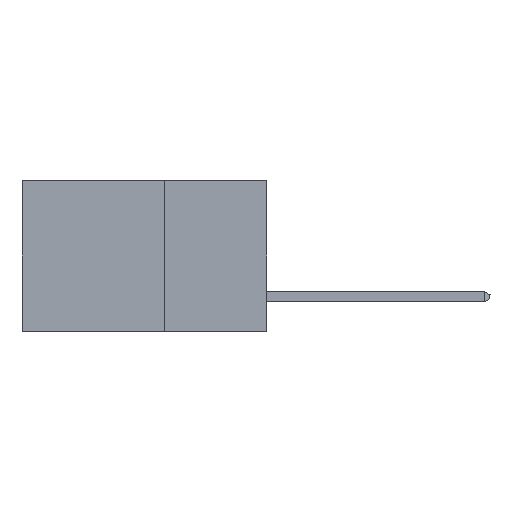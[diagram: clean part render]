
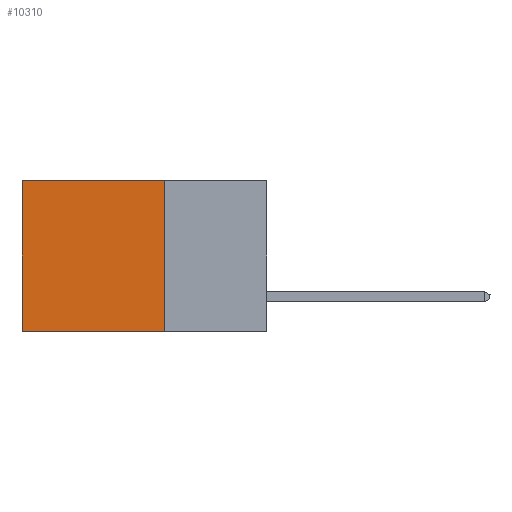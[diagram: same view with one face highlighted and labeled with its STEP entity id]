
A CAD part, left-side view. The second image highlights one B-rep face of the part: STEP entity #10310.
In plain terms, the highlighted planar face has unit normal (-1, 0, 0).
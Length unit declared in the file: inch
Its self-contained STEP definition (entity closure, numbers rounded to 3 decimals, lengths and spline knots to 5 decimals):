
#610 = DIRECTION ( 'NONE',  ( 0., 0., -1. ) ) ;
#1296 = DIRECTION ( 'NONE',  ( 0., 1., 0. ) ) ;
#2997 = VERTEX_POINT ( 'NONE', #9254 ) ;
#3618 = CARTESIAN_POINT ( 'NONE',  ( 0.2875, 0.6, 0. ) ) ;
#3729 = CARTESIAN_POINT ( 'NONE',  ( 0.2875, 0.25, 0. ) ) ;
#5821 = PLANE ( 'NONE',  #21816 ) ;
#5862 = CARTESIAN_POINT ( 'NONE',  ( 0.2875, 0.6, 0. ) ) ;
#5913 = LINE ( 'NONE', #28726, #9080 ) ;
#6193 = CARTESIAN_POINT ( 'NONE',  ( 0.2875, 0.25, 0. ) ) ;
#8017 = ORIENTED_EDGE ( 'NONE', *, *, #26183, .T. ) ;
#9080 = VECTOR ( 'NONE', #26464, 39.37008 ) ;
#9254 = CARTESIAN_POINT ( 'NONE',  ( 0.2875, 0.25, -0.37 ) ) ;
#9255 = CARTESIAN_POINT ( 'NONE',  ( 0.2875, 0.6, -0.37 ) ) ;
#9901 = VECTOR ( 'NONE', #19929, 39.37008 ) ;
#10310 = ADVANCED_FACE ( 'NONE', ( #14780 ), #5821, .F. ) ;
#11364 = VERTEX_POINT ( 'NONE', #3729 ) ;
#13336 = VECTOR ( 'NONE', #28371, 39.37008 ) ;
#14574 = LINE ( 'NONE', #3618, #13336 ) ;
#14780 = FACE_OUTER_BOUND ( 'NONE', #30407, .T. ) ;
#15592 = EDGE_CURVE ( 'NONE', #2997, #28234, #5913, .T. ) ;
#15594 = CARTESIAN_POINT ( 'NONE',  ( 0.2875, 0.25, 0. ) ) ;
#17346 = CARTESIAN_POINT ( 'NONE',  ( 0.2875, 0.25, 0. ) ) ;
#17955 = LINE ( 'NONE', #6193, #22240 ) ;
#19929 = DIRECTION ( 'NONE',  ( 0., 0., -1. ) ) ;
#21816 = AXIS2_PLACEMENT_3D ( 'NONE', #15594, #30573, #610 ) ;
#22240 = VECTOR ( 'NONE', #1296, 39.37008 ) ;
#23513 = VERTEX_POINT ( 'NONE', #5862 ) ;
#25697 = ORIENTED_EDGE ( 'NONE', *, *, #28062, .T. ) ;
#26183 = EDGE_CURVE ( 'NONE', #23513, #28234, #14574, .T. ) ;
#26464 = DIRECTION ( 'NONE',  ( 0., 1., 0. ) ) ;
#27023 = EDGE_CURVE ( 'NONE', #11364, #2997, #27738, .T. ) ;
#27738 = LINE ( 'NONE', #17346, #9901 ) ;
#28062 = EDGE_CURVE ( 'NONE', #11364, #23513, #17955, .T. ) ;
#28234 = VERTEX_POINT ( 'NONE', #9255 ) ;
#28371 = DIRECTION ( 'NONE',  ( 0., 0., -1. ) ) ;
#28726 = CARTESIAN_POINT ( 'NONE',  ( 0.2875, 0.25, -0.37 ) ) ;
#28901 = ORIENTED_EDGE ( 'NONE', *, *, #15592, .F. ) ;
#29964 = ORIENTED_EDGE ( 'NONE', *, *, #27023, .F. ) ;
#30407 = EDGE_LOOP ( 'NONE', ( #8017, #28901, #29964, #25697 ) ) ;
#30573 = DIRECTION ( 'NONE',  ( 1., 0., 0. ) ) ;
